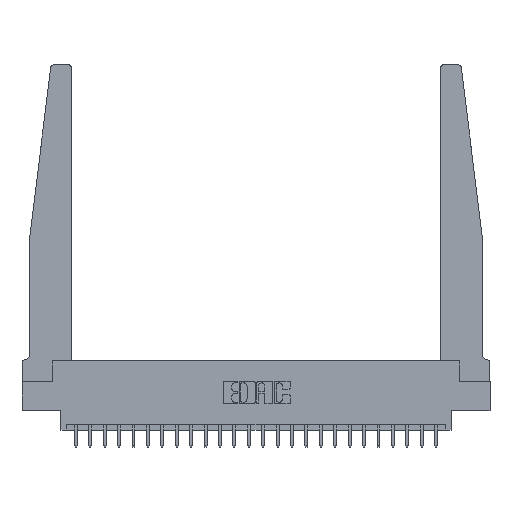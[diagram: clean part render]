
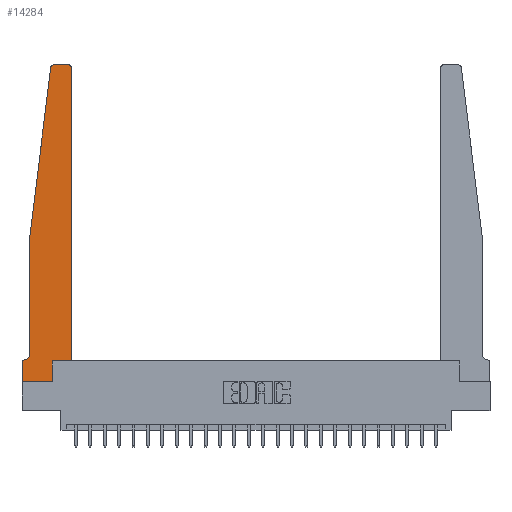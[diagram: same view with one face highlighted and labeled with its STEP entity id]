
A CAD part, top view. The second image highlights one B-rep face of the part: STEP entity #14284.
In plain terms, the highlighted planar face has unit normal (0, 0, 1).
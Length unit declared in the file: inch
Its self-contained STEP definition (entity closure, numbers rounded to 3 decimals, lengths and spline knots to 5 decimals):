
#265 = CARTESIAN_POINT ( 'NONE',  ( 0., 0.1875, 0.37 ) ) ;
#610 = EDGE_CURVE ( 'NONE', #895, #3083, #19677, .T. ) ;
#758 = CARTESIAN_POINT ( 'NONE',  ( 0., 0., 0.37 ) ) ;
#895 = VERTEX_POINT ( 'NONE', #18925 ) ;
#911 = ORIENTED_EDGE ( 'NONE', *, *, #17710, .T. ) ;
#920 = VERTEX_POINT ( 'NONE', #2275 ) ;
#1178 = VECTOR ( 'NONE', #2326, 39.37008 ) ;
#1536 = CIRCLE ( 'NONE', #18570, 0.03 ) ;
#2275 = CARTESIAN_POINT ( 'NONE',  ( 0., 0., 0.37 ) ) ;
#2326 = DIRECTION ( 'NONE',  ( 0., 1., 0. ) ) ;
#2575 = CIRCLE ( 'NONE', #7739, 0.05 ) ;
#2586 = CARTESIAN_POINT ( 'NONE',  ( 0., 0.1875, 0.37 ) ) ;
#2759 = ORIENTED_EDGE ( 'NONE', *, *, #7726, .T. ) ;
#2805 = VECTOR ( 'NONE', #13307, 39.37008 ) ;
#3083 = VERTEX_POINT ( 'NONE', #18771 ) ;
#3256 = CARTESIAN_POINT ( 'NONE',  ( 0.065, 0.1875, 0.37 ) ) ;
#3425 = VECTOR ( 'NONE', #22786, 39.37008 ) ;
#4070 = VERTEX_POINT ( 'NONE', #13759 ) ;
#4095 = VERTEX_POINT ( 'NONE', #23282 ) ;
#4863 = CARTESIAN_POINT ( 'NONE',  ( 0.015, 0.1875, 0.37 ) ) ;
#4951 = CARTESIAN_POINT ( 'NONE',  ( 0.425, 2.72, 0.37 ) ) ;
#5040 = CARTESIAN_POINT ( 'NONE',  ( 0.2605, 0.18, 0.37 ) ) ;
#5254 = AXIS2_PLACEMENT_3D ( 'NONE', #265, #17647, #11945 ) ;
#5285 = VERTEX_POINT ( 'NONE', #4951 ) ;
#5694 = CARTESIAN_POINT ( 'NONE',  ( 0., 0., 0.37 ) ) ;
#5882 = VERTEX_POINT ( 'NONE', #21867 ) ;
#5928 = LINE ( 'NONE', #5694, #2805 ) ;
#5943 = CARTESIAN_POINT ( 'NONE',  ( 0.015, 0.2375, 0.37 ) ) ;
#6813 = LINE ( 'NONE', #758, #7715 ) ;
#7102 = EDGE_CURVE ( 'NONE', #5882, #24479, #7667, .T. ) ;
#7188 = DIRECTION ( 'NONE',  ( 0., 0., 1. ) ) ;
#7220 = DIRECTION ( 'NONE',  ( -1., 0., 0. ) ) ;
#7359 = VERTEX_POINT ( 'NONE', #20639 ) ;
#7397 = ORIENTED_EDGE ( 'NONE', *, *, #610, .T. ) ;
#7667 = LINE ( 'NONE', #9758, #3425 ) ;
#7715 = VECTOR ( 'NONE', #23706, 39.37008 ) ;
#7726 = EDGE_CURVE ( 'NONE', #22615, #4095, #9827, .T. ) ;
#7739 = AXIS2_PLACEMENT_3D ( 'NONE', #5943, #23210, #13817 ) ;
#8202 = PLANE ( 'NONE',  #5254 ) ;
#9403 = AXIS2_PLACEMENT_3D ( 'NONE', #17868, #12292, #12537 ) ;
#9758 = CARTESIAN_POINT ( 'NONE',  ( 0.065, 1.25, 0.37 ) ) ;
#9826 = DIRECTION ( 'NONE',  ( 1., 0., 0. ) ) ;
#9827 = LINE ( 'NONE', #11834, #11979 ) ;
#10222 = EDGE_CURVE ( 'NONE', #3083, #7359, #11712, .T. ) ;
#11659 = LINE ( 'NONE', #19303, #16999 ) ;
#11712 = LINE ( 'NONE', #19233, #24018 ) ;
#11834 = CARTESIAN_POINT ( 'NONE',  ( 0.25, 2.75, 0.37 ) ) ;
#11945 = DIRECTION ( 'NONE',  ( 1., 0., 0. ) ) ;
#11979 = VECTOR ( 'NONE', #21593, 39.37008 ) ;
#12292 = DIRECTION ( 'NONE',  ( 0., 0., 1. ) ) ;
#12537 = DIRECTION ( 'NONE',  ( 1., 0., 0. ) ) ;
#13302 = EDGE_CURVE ( 'NONE', #24479, #23556, #2575, .T. ) ;
#13307 = DIRECTION ( 'NONE',  ( 0., -1., 0. ) ) ;
#13747 = EDGE_LOOP ( 'NONE', ( #2759, #911, #19519, #20454, #16185, #21200, #23513, #14996, #7397, #13756, #15615, #13749 ) ) ;
#13749 = ORIENTED_EDGE ( 'NONE', *, *, #14633, .T. ) ;
#13756 = ORIENTED_EDGE ( 'NONE', *, *, #10222, .T. ) ;
#13759 = CARTESIAN_POINT ( 'NONE',  ( 0.24675, 2.72367, 0.37 ) ) ;
#13786 = CARTESIAN_POINT ( 'NONE',  ( 0.425, 0.18, 0.37 ) ) ;
#13817 = DIRECTION ( 'NONE',  ( -1., 0., 0. ) ) ;
#14284 = ADVANCED_FACE ( 'NONE', ( #17174 ), #8202, .T. ) ;
#14409 = EDGE_CURVE ( 'NONE', #920, #895, #6813, .T. ) ;
#14633 = EDGE_CURVE ( 'NONE', #5285, #22615, #1536, .T. ) ;
#14834 = LINE ( 'NONE', #3256, #24448 ) ;
#14996 = ORIENTED_EDGE ( 'NONE', *, *, #14409, .T. ) ;
#15031 = CARTESIAN_POINT ( 'NONE',  ( 0.065, 0.2375, 0.37 ) ) ;
#15615 = ORIENTED_EDGE ( 'NONE', *, *, #19526, .T. ) ;
#15868 = CARTESIAN_POINT ( 'NONE',  ( 0.395, 2.75, 0.37 ) ) ;
#15889 = LINE ( 'NONE', #13786, #1178 ) ;
#16185 = ORIENTED_EDGE ( 'NONE', *, *, #13302, .T. ) ;
#16711 = VECTOR ( 'NONE', #18088, 39.37008 ) ;
#16977 = CIRCLE ( 'NONE', #9403, 0.03 ) ;
#16999 = VECTOR ( 'NONE', #19429, 39.37008 ) ;
#17174 = FACE_OUTER_BOUND ( 'NONE', #13747, .T. ) ;
#17402 = EDGE_CURVE ( 'NONE', #23556, #22205, #14834, .T. ) ;
#17647 = DIRECTION ( 'NONE',  ( 0., 0., 1. ) ) ;
#17710 = EDGE_CURVE ( 'NONE', #4095, #4070, #16977, .T. ) ;
#17868 = CARTESIAN_POINT ( 'NONE',  ( 0.27653, 2.72, 0.37 ) ) ;
#18088 = DIRECTION ( 'NONE',  ( 0., 1., 0. ) ) ;
#18257 = EDGE_CURVE ( 'NONE', #4070, #5882, #11659, .T. ) ;
#18570 = AXIS2_PLACEMENT_3D ( 'NONE', #22322, #7188, #22442 ) ;
#18771 = CARTESIAN_POINT ( 'NONE',  ( 0.2605, 0.18, 0.37 ) ) ;
#18925 = CARTESIAN_POINT ( 'NONE',  ( 0.2605, 0., 0.37 ) ) ;
#19233 = CARTESIAN_POINT ( 'NONE',  ( 0.425, 0.18, 0.37 ) ) ;
#19303 = CARTESIAN_POINT ( 'NONE',  ( 0.065, 1.25, 0.37 ) ) ;
#19429 = DIRECTION ( 'NONE',  ( -0.122, -0.992, 0. ) ) ;
#19519 = ORIENTED_EDGE ( 'NONE', *, *, #18257, .T. ) ;
#19526 = EDGE_CURVE ( 'NONE', #7359, #5285, #15889, .T. ) ;
#19677 = LINE ( 'NONE', #5040, #16711 ) ;
#20454 = ORIENTED_EDGE ( 'NONE', *, *, #7102, .T. ) ;
#20639 = CARTESIAN_POINT ( 'NONE',  ( 0.425, 0.18, 0.37 ) ) ;
#21200 = ORIENTED_EDGE ( 'NONE', *, *, #17402, .T. ) ;
#21593 = DIRECTION ( 'NONE',  ( -1., 0., 0. ) ) ;
#21867 = CARTESIAN_POINT ( 'NONE',  ( 0.065, 1.25, 0.37 ) ) ;
#22205 = VERTEX_POINT ( 'NONE', #2586 ) ;
#22322 = CARTESIAN_POINT ( 'NONE',  ( 0.395, 2.72, 0.37 ) ) ;
#22442 = DIRECTION ( 'NONE',  ( 1., 0., 0. ) ) ;
#22615 = VERTEX_POINT ( 'NONE', #15868 ) ;
#22786 = DIRECTION ( 'NONE',  ( 0., -1., 0. ) ) ;
#23141 = EDGE_CURVE ( 'NONE', #22205, #920, #5928, .T. ) ;
#23210 = DIRECTION ( 'NONE',  ( 0., 0., -1. ) ) ;
#23282 = CARTESIAN_POINT ( 'NONE',  ( 0.27653, 2.75, 0.37 ) ) ;
#23513 = ORIENTED_EDGE ( 'NONE', *, *, #23141, .T. ) ;
#23556 = VERTEX_POINT ( 'NONE', #4863 ) ;
#23706 = DIRECTION ( 'NONE',  ( 1., 0., 0. ) ) ;
#24018 = VECTOR ( 'NONE', #9826, 39.37008 ) ;
#24448 = VECTOR ( 'NONE', #7220, 39.37008 ) ;
#24479 = VERTEX_POINT ( 'NONE', #15031 ) ;
